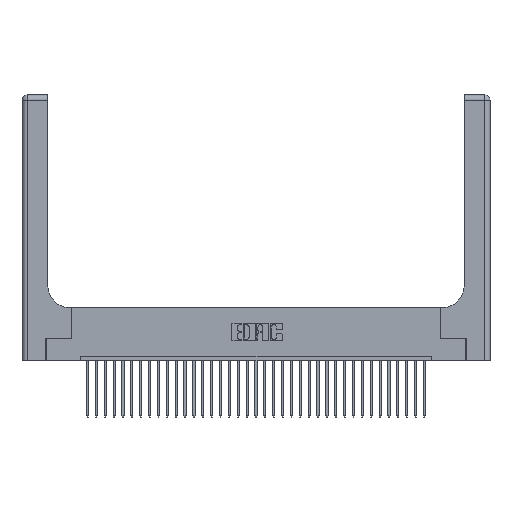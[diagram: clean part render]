
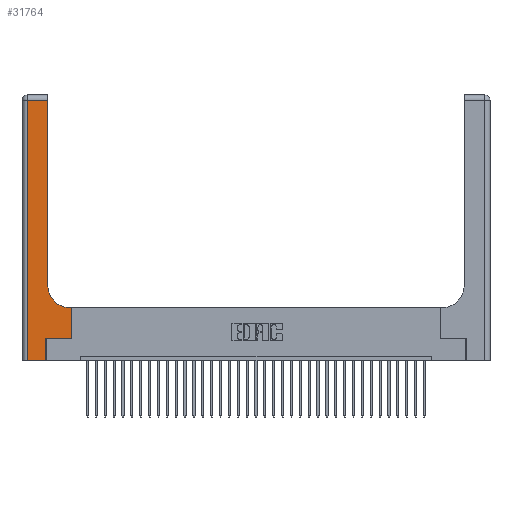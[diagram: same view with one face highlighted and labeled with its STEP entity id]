
A CAD part, top view. The second image highlights one B-rep face of the part: STEP entity #31764.
In plain terms, the highlighted planar face has unit normal (0, 0, 1).
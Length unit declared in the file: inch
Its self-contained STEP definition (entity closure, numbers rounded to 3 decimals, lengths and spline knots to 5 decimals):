
#41 = CARTESIAN_POINT ( 'NONE',  ( 0.5585, 0.25, 0.37 ) ) ;
#663 = CARTESIAN_POINT ( 'NONE',  ( 0.5415, 0.6, 0.37 ) ) ;
#2147 = VERTEX_POINT ( 'NONE', #16570 ) ;
#2287 = VERTEX_POINT ( 'NONE', #3983 ) ;
#2964 = ORIENTED_EDGE ( 'NONE', *, *, #34935, .T. ) ;
#3040 = FACE_OUTER_BOUND ( 'NONE', #18451, .T. ) ;
#3544 = EDGE_CURVE ( 'NONE', #30055, #16839, #8108, .T. ) ;
#3983 = CARTESIAN_POINT ( 'NONE',  ( 0.269, 0.25, 0.37 ) ) ;
#4376 = VERTEX_POINT ( 'NONE', #29640 ) ;
#4590 = VERTEX_POINT ( 'NONE', #29736 ) ;
#5036 = LINE ( 'NONE', #9657, #21870 ) ;
#6033 = VECTOR ( 'NONE', #15499, 39.37008 ) ;
#6194 = PLANE ( 'NONE',  #7649 ) ;
#6306 = LINE ( 'NONE', #9511, #19765 ) ;
#6348 = ORIENTED_EDGE ( 'NONE', *, *, #3544, .T. ) ;
#6771 = DIRECTION ( 'NONE',  ( 0., 0., -1. ) ) ;
#6780 = VERTEX_POINT ( 'NONE', #41 ) ;
#7044 = DIRECTION ( 'NONE',  ( -1., 0., 0. ) ) ;
#7099 = CARTESIAN_POINT ( 'NONE',  ( 0.5585, 0.25, 0.37 ) ) ;
#7397 = LINE ( 'NONE', #9373, #6033 ) ;
#7649 = AXIS2_PLACEMENT_3D ( 'NONE', #25167, #25038, #14134 ) ;
#8108 = LINE ( 'NONE', #14178, #34703 ) ;
#8443 = VECTOR ( 'NONE', #11323, 39.37008 ) ;
#8947 = CARTESIAN_POINT ( 'NONE',  ( 0.269, 0., 0.37 ) ) ;
#9373 = CARTESIAN_POINT ( 'NONE',  ( 0., 0., 0.37 ) ) ;
#9487 = DIRECTION ( 'NONE',  ( 1., 0., 0. ) ) ;
#9511 = CARTESIAN_POINT ( 'NONE',  ( 0., 2.94, 0.37 ) ) ;
#9531 = CARTESIAN_POINT ( 'NONE',  ( 0.5585, 0.6, 0.37 ) ) ;
#9657 = CARTESIAN_POINT ( 'NONE',  ( 0.269, 0.25, 0.37 ) ) ;
#9929 = DIRECTION ( 'NONE',  ( 0., 1., 0. ) ) ;
#11103 = EDGE_CURVE ( 'NONE', #2147, #2287, #26305, .T. ) ;
#11176 = ORIENTED_EDGE ( 'NONE', *, *, #16110, .T. ) ;
#11323 = DIRECTION ( 'NONE',  ( 0., 1., 0. ) ) ;
#12361 = DIRECTION ( 'NONE',  ( 1., 0., 0. ) ) ;
#13545 = VECTOR ( 'NONE', #31851, 39.37008 ) ;
#14134 = DIRECTION ( 'NONE',  ( -1., 0., 0. ) ) ;
#14171 = EDGE_CURVE ( 'NONE', #2287, #6780, #5036, .T. ) ;
#14178 = CARTESIAN_POINT ( 'NONE',  ( 0.2915, 0.6, 0.37 ) ) ;
#14304 = DIRECTION ( 'NONE',  ( -1., 0., 0. ) ) ;
#14309 = CARTESIAN_POINT ( 'NONE',  ( 0.2915, 3., 0.37 ) ) ;
#14397 = LINE ( 'NONE', #31966, #13545 ) ;
#14788 = AXIS2_PLACEMENT_3D ( 'NONE', #15159, #6771, #9487 ) ;
#15159 = CARTESIAN_POINT ( 'NONE',  ( 0.5415, 0.85, 0.37 ) ) ;
#15499 = DIRECTION ( 'NONE',  ( 1., 0., 0. ) ) ;
#16110 = EDGE_CURVE ( 'NONE', #16839, #19164, #16631, .T. ) ;
#16192 = VERTEX_POINT ( 'NONE', #20637 ) ;
#16570 = CARTESIAN_POINT ( 'NONE',  ( 0.269, 0., 0.37 ) ) ;
#16631 = CIRCLE ( 'NONE', #14788, 0.25 ) ;
#16839 = VERTEX_POINT ( 'NONE', #663 ) ;
#16943 = LINE ( 'NONE', #7099, #22898 ) ;
#17065 = EDGE_CURVE ( 'NONE', #4590, #2147, #7397, .T. ) ;
#17326 = LINE ( 'NONE', #14309, #8443 ) ;
#17570 = DIRECTION ( 'NONE',  ( 0., 1., 0. ) ) ;
#17932 = ORIENTED_EDGE ( 'NONE', *, *, #11103, .T. ) ;
#18326 = EDGE_CURVE ( 'NONE', #6780, #30055, #16943, .T. ) ;
#18451 = EDGE_LOOP ( 'NONE', ( #21927, #2964, #33231, #34769, #17932, #30088, #32172, #6348, #11176 ) ) ;
#19164 = VERTEX_POINT ( 'NONE', #26211 ) ;
#19765 = VECTOR ( 'NONE', #7044, 39.37008 ) ;
#20637 = CARTESIAN_POINT ( 'NONE',  ( 0.06, 2.94, 0.37 ) ) ;
#21870 = VECTOR ( 'NONE', #12361, 39.37008 ) ;
#21927 = ORIENTED_EDGE ( 'NONE', *, *, #33569, .T. ) ;
#22898 = VECTOR ( 'NONE', #9929, 39.37008 ) ;
#25038 = DIRECTION ( 'NONE',  ( 0., 0., -1. ) ) ;
#25167 = CARTESIAN_POINT ( 'NONE',  ( 0., 3., 0.37 ) ) ;
#25906 = VECTOR ( 'NONE', #17570, 39.37008 ) ;
#26211 = CARTESIAN_POINT ( 'NONE',  ( 0.2915, 0.85, 0.37 ) ) ;
#26305 = LINE ( 'NONE', #8947, #25906 ) ;
#29640 = CARTESIAN_POINT ( 'NONE',  ( 0.2915, 2.94, 0.37 ) ) ;
#29736 = CARTESIAN_POINT ( 'NONE',  ( 0.06, 0., 0.37 ) ) ;
#30055 = VERTEX_POINT ( 'NONE', #9531 ) ;
#30088 = ORIENTED_EDGE ( 'NONE', *, *, #14171, .T. ) ;
#31764 = ADVANCED_FACE ( 'NONE', ( #3040 ), #6194, .F. ) ;
#31851 = DIRECTION ( 'NONE',  ( 0., -1., 0. ) ) ;
#31966 = CARTESIAN_POINT ( 'NONE',  ( 0.06, 3., 0.37 ) ) ;
#32172 = ORIENTED_EDGE ( 'NONE', *, *, #18326, .T. ) ;
#33231 = ORIENTED_EDGE ( 'NONE', *, *, #33878, .T. ) ;
#33569 = EDGE_CURVE ( 'NONE', #19164, #4376, #17326, .T. ) ;
#33878 = EDGE_CURVE ( 'NONE', #16192, #4590, #14397, .T. ) ;
#34703 = VECTOR ( 'NONE', #14304, 39.37008 ) ;
#34769 = ORIENTED_EDGE ( 'NONE', *, *, #17065, .T. ) ;
#34935 = EDGE_CURVE ( 'NONE', #4376, #16192, #6306, .T. ) ;
